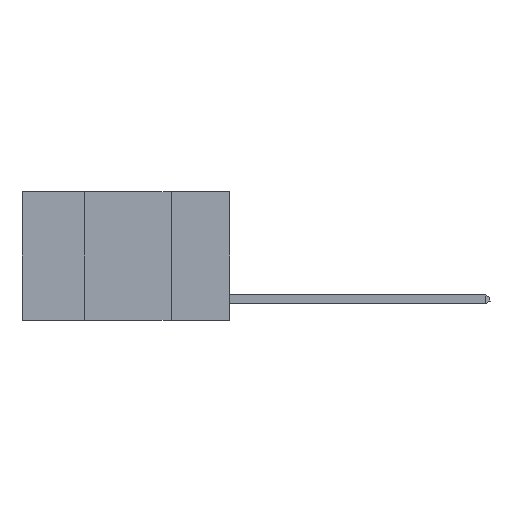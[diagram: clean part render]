
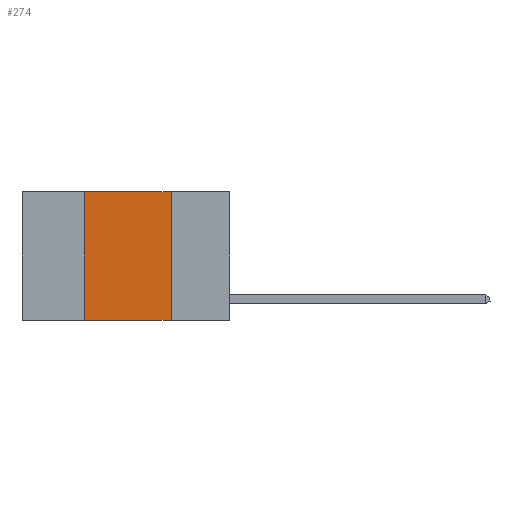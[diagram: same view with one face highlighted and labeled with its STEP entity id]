
A CAD part, left-side view. The second image highlights one B-rep face of the part: STEP entity #274.
In plain terms, the highlighted planar face has unit normal (-1, 0, 0).
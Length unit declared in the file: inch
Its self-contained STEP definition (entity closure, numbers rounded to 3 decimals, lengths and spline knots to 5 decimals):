
#274 = ADVANCED_FACE ( 'NONE', ( #8937 ), #872, .F. ) ;
#360 = CARTESIAN_POINT ( 'NONE',  ( 0., 0.42, 0. ) ) ;
#696 = CARTESIAN_POINT ( 'NONE',  ( 0., 0.6, -0.37 ) ) ;
#790 = DIRECTION ( 'NONE',  ( 1., 0., 0. ) ) ;
#872 = PLANE ( 'NONE',  #3096 ) ;
#1290 = CARTESIAN_POINT ( 'NONE',  ( 0., 0.17, 0. ) ) ;
#1897 = EDGE_CURVE ( 'NONE', #9818, #12949, #13526, .T. ) ;
#2849 = EDGE_CURVE ( 'NONE', #12949, #13554, #11530, .T. ) ;
#3096 = AXIS2_PLACEMENT_3D ( 'NONE', #5510, #790, #10153 ) ;
#3136 = DIRECTION ( 'NONE',  ( 0., 0., 1. ) ) ;
#3565 = DIRECTION ( 'NONE',  ( 0., 0., -1. ) ) ;
#4697 = VERTEX_POINT ( 'NONE', #11539 ) ;
#5399 = LINE ( 'NONE', #696, #14899 ) ;
#5510 = CARTESIAN_POINT ( 'NONE',  ( 0., 0.6, 0. ) ) ;
#5763 = CARTESIAN_POINT ( 'NONE',  ( 0., 0.6, 0. ) ) ;
#7229 = CARTESIAN_POINT ( 'NONE',  ( 0., 0.17, 0. ) ) ;
#7998 = EDGE_CURVE ( 'NONE', #13554, #4697, #8357, .T. ) ;
#8357 = LINE ( 'NONE', #7229, #8841 ) ;
#8449 = ORIENTED_EDGE ( 'NONE', *, *, #9042, .T. ) ;
#8621 = EDGE_LOOP ( 'NONE', ( #13092, #9037, #12756, #8449 ) ) ;
#8841 = VECTOR ( 'NONE', #3565, 39.37008 ) ;
#8937 = FACE_OUTER_BOUND ( 'NONE', #8621, .T. ) ;
#9037 = ORIENTED_EDGE ( 'NONE', *, *, #2849, .F. ) ;
#9042 = EDGE_CURVE ( 'NONE', #9818, #4697, #5399, .T. ) ;
#9818 = VERTEX_POINT ( 'NONE', #14292 ) ;
#10153 = DIRECTION ( 'NONE',  ( 0., 0., -1. ) ) ;
#10397 = DIRECTION ( 'NONE',  ( 0., -1., 0. ) ) ;
#11530 = LINE ( 'NONE', #5763, #11566 ) ;
#11539 = CARTESIAN_POINT ( 'NONE',  ( 0., 0.17, -0.37 ) ) ;
#11566 = VECTOR ( 'NONE', #10397, 39.37008 ) ;
#11777 = VECTOR ( 'NONE', #3136, 39.37008 ) ;
#12314 = DIRECTION ( 'NONE',  ( 0., -1., 0. ) ) ;
#12394 = CARTESIAN_POINT ( 'NONE',  ( 0., 0.42, 0. ) ) ;
#12756 = ORIENTED_EDGE ( 'NONE', *, *, #1897, .F. ) ;
#12949 = VERTEX_POINT ( 'NONE', #360 ) ;
#13092 = ORIENTED_EDGE ( 'NONE', *, *, #7998, .F. ) ;
#13526 = LINE ( 'NONE', #12394, #11777 ) ;
#13554 = VERTEX_POINT ( 'NONE', #1290 ) ;
#14292 = CARTESIAN_POINT ( 'NONE',  ( 0., 0.42, -0.37 ) ) ;
#14899 = VECTOR ( 'NONE', #12314, 39.37008 ) ;
